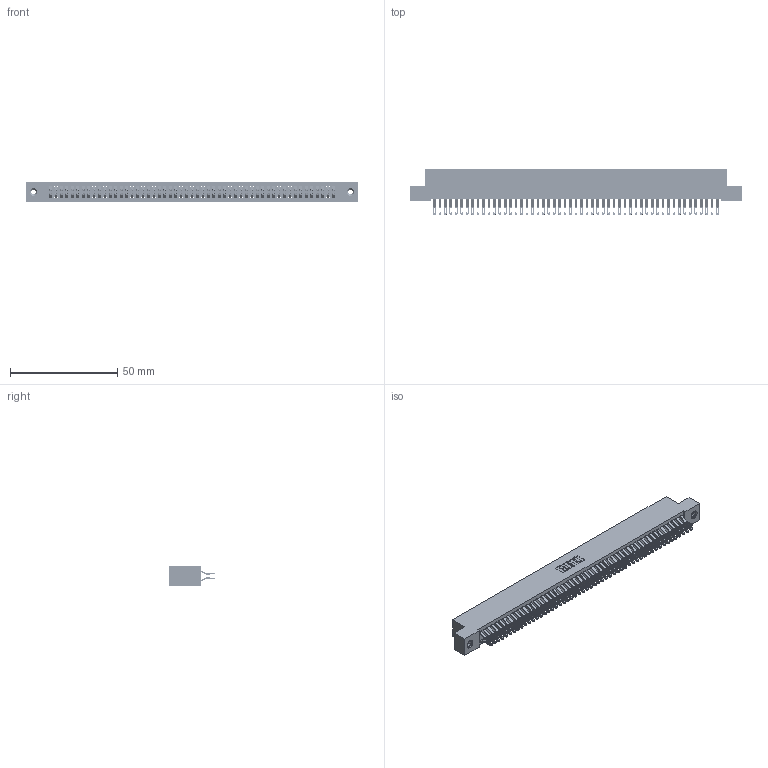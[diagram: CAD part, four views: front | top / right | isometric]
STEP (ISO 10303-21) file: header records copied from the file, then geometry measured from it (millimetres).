
FILE_DESCRIPTION (( 'STEP AP203' ), '1' );
FILE_NAME ('342-106-555-208.STEP', '2018-08-14T07:11:17', ( '' ), ( '' ), 'SwSTEP 2.0', 'SolidWorks 2016', '' );
FILE_SCHEMA (( 'CONFIG_CONTROL_DESIGN' ));
Length unit declared in the file: inch
Products named in the file (4): 342 Part_TI; 345-292-001_555 Tail; 345-250-001_345-250-003-102; 342-106-555-208
Assembly tree (109 placements, depth 2):
  342-106-555-208
    342 Part_TI
    345-292-001_555 Tail  x106
    345-250-001_345-250-003-102  x2
Bounding box: 154.94 x 21.47 x 9.4 mm (x, y, z)
Volume: 14262.3 mm3; surface area: 24522.4 mm2
Topology: 109 solids, 109 shells, 6318 faces, 19833 edges, 13214 vertices
Faces by surface type: plane 3702, cylinder 2600, cone 12, torus 4
Entity records: 34054 total; most frequent: CARTESIAN_POINT 5647, ORIENTED_EDGE 5546, DIRECTION 4807, EDGE_CURVE 2773, LINE 2605, VECTOR 2605, VERTEX_POINT 1844, AXIS2_PLACEMENT_3D 1101
